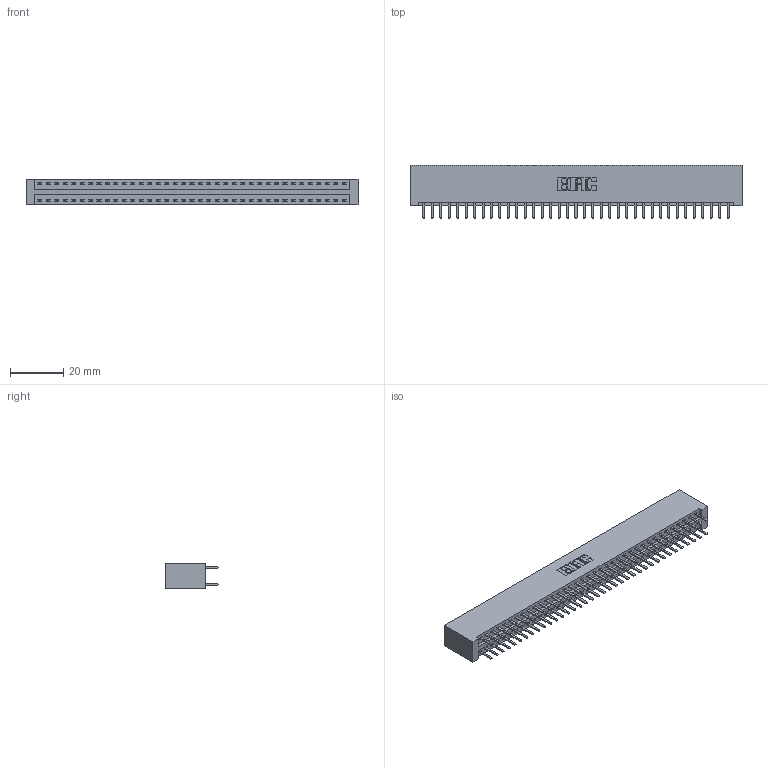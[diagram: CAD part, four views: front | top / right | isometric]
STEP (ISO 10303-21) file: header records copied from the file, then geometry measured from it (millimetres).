
FILE_DESCRIPTION (( 'STEP AP203' ), '1' );
FILE_NAME ('346-074-520-201.STEP', '2018-08-29T01:52:04', ( '' ), ( '' ), 'SwSTEP 2.0', 'SolidWorks 2016', '' );
FILE_SCHEMA (( 'CONFIG_CONTROL_DESIGN' ));
Length unit declared in the file: inch
Products named in the file (3): 346 Part_No Mounting Lugs; 345-292-001_345-293-120; 346-074-520-201
Assembly tree (75 placements, depth 2):
  346-074-520-201
    346 Part_No Mounting Lugs
    345-292-001_345-293-120  x74
Bounding box: 124.71 x 20.02 x 9.4 mm (x, y, z)
Volume: 12663.1 mm3; surface area: 17414.6 mm2
Topology: 75 solids, 75 shells, 4258 faces, 12367 edges, 8046 vertices
Faces by surface type: plane 2810, cylinder 1448
Entity records: 24657 total; most frequent: CARTESIAN_POINT 4080, ORIENTED_EDGE 4002, DIRECTION 3629, EDGE_CURVE 2001, VECTOR 1725, LINE 1725, VERTEX_POINT 1330, AXIS2_PLACEMENT_3D 952
